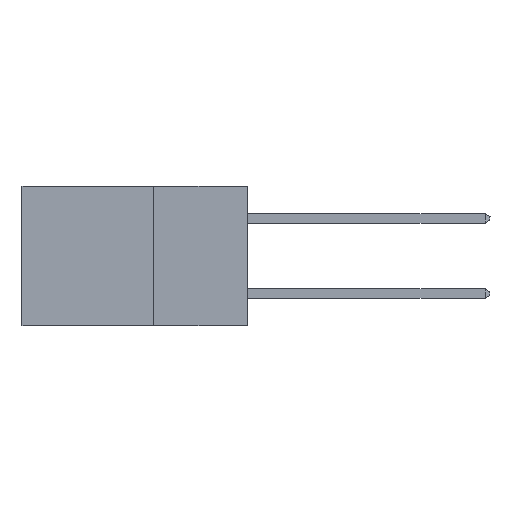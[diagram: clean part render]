
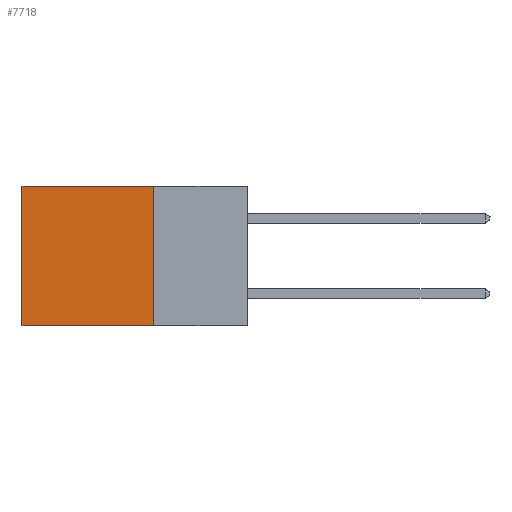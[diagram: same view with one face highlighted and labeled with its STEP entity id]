
A CAD part, left-side view. The second image highlights one B-rep face of the part: STEP entity #7718.
In plain terms, the highlighted planar face has unit normal (-1, 0, 0).
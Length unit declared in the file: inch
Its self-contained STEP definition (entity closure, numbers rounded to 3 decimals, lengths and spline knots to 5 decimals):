
#546 = CARTESIAN_POINT ( 'NONE',  ( 0.298, 0.6, 0. ) ) ;
#551 = ORIENTED_EDGE ( 'NONE', *, *, #18811, .T. ) ;
#2998 = DIRECTION ( 'NONE',  ( 0., 0., -1. ) ) ;
#4047 = VERTEX_POINT ( 'NONE', #7658 ) ;
#5331 = CARTESIAN_POINT ( 'NONE',  ( 0.298, 0.6, 0. ) ) ;
#7105 = DIRECTION ( 'NONE',  ( 1., 0., 0. ) ) ;
#7658 = CARTESIAN_POINT ( 'NONE',  ( 0.298, 0.25, -0.37 ) ) ;
#7718 = ADVANCED_FACE ( 'NONE', ( #23165 ), #21138, .F. ) ;
#8014 = EDGE_LOOP ( 'NONE', ( #551, #24544, #12136, #12312 ) ) ;
#8096 = VERTEX_POINT ( 'NONE', #17716 ) ;
#9683 = DIRECTION ( 'NONE',  ( 0., 1., 0. ) ) ;
#11571 = VECTOR ( 'NONE', #9683, 39.37008 ) ;
#12136 = ORIENTED_EDGE ( 'NONE', *, *, #27412, .F. ) ;
#12312 = ORIENTED_EDGE ( 'NONE', *, *, #21743, .T. ) ;
#12715 = LINE ( 'NONE', #25217, #17501 ) ;
#13184 = VERTEX_POINT ( 'NONE', #17147 ) ;
#14801 = VECTOR ( 'NONE', #2998, 39.37008 ) ;
#15465 = AXIS2_PLACEMENT_3D ( 'NONE', #30471, #7105, #23510 ) ;
#15529 = LINE ( 'NONE', #546, #14801 ) ;
#16365 = VECTOR ( 'NONE', #29895, 39.37008 ) ;
#16474 = EDGE_CURVE ( 'NONE', #4047, #8096, #12715, .T. ) ;
#17147 = CARTESIAN_POINT ( 'NONE',  ( 0.298, 0.25, 0. ) ) ;
#17501 = VECTOR ( 'NONE', #18314, 39.37008 ) ;
#17716 = CARTESIAN_POINT ( 'NONE',  ( 0.298, 0.6, -0.37 ) ) ;
#18314 = DIRECTION ( 'NONE',  ( 0., 1., 0. ) ) ;
#18784 = VERTEX_POINT ( 'NONE', #5331 ) ;
#18811 = EDGE_CURVE ( 'NONE', #18784, #8096, #15529, .T. ) ;
#21138 = PLANE ( 'NONE',  #15465 ) ;
#21743 = EDGE_CURVE ( 'NONE', #13184, #18784, #24062, .T. ) ;
#23165 = FACE_OUTER_BOUND ( 'NONE', #8014, .T. ) ;
#23510 = DIRECTION ( 'NONE',  ( 0., 0., -1. ) ) ;
#24062 = LINE ( 'NONE', #26208, #11571 ) ;
#24544 = ORIENTED_EDGE ( 'NONE', *, *, #16474, .F. ) ;
#25217 = CARTESIAN_POINT ( 'NONE',  ( 0.298, 0.25, -0.37 ) ) ;
#26208 = CARTESIAN_POINT ( 'NONE',  ( 0.298, 0.25, 0. ) ) ;
#27412 = EDGE_CURVE ( 'NONE', #13184, #4047, #28180, .T. ) ;
#27575 = CARTESIAN_POINT ( 'NONE',  ( 0.298, 0.25, 0. ) ) ;
#28180 = LINE ( 'NONE', #27575, #16365 ) ;
#29895 = DIRECTION ( 'NONE',  ( 0., 0., -1. ) ) ;
#30471 = CARTESIAN_POINT ( 'NONE',  ( 0.298, 0.25, 0. ) ) ;
